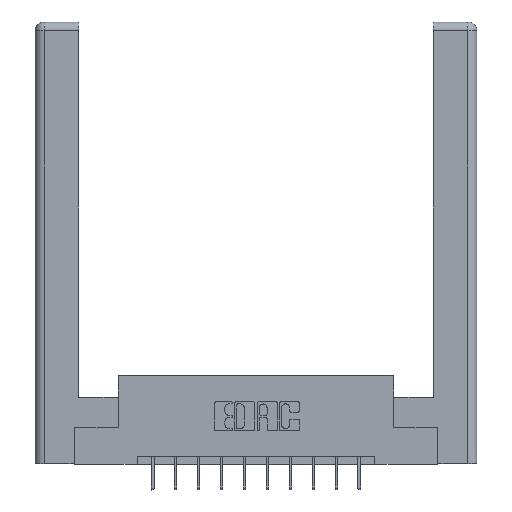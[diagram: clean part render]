
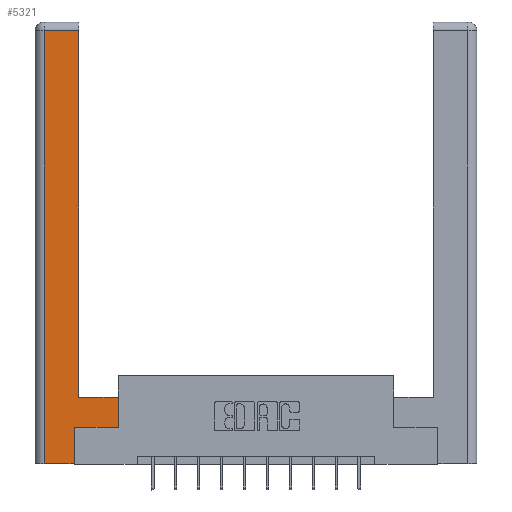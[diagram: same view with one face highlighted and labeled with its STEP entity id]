
A CAD part, top view. The second image highlights one B-rep face of the part: STEP entity #5321.
In plain terms, the highlighted planar face has unit normal (0, 0, 1).
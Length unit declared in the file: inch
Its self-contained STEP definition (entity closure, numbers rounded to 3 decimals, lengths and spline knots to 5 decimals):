
#81 = CARTESIAN_POINT ( 'NONE',  ( 0.0615, 2.94, 0. ) ) ;
#322 = CARTESIAN_POINT ( 'NONE',  ( 0., 0., 0. ) ) ;
#514 = DIRECTION ( 'NONE',  ( -1., 0., 0. ) ) ;
#683 = VERTEX_POINT ( 'NONE', #6908 ) ;
#721 = EDGE_CURVE ( 'NONE', #13895, #5554, #6565, .T. ) ;
#942 = EDGE_CURVE ( 'NONE', #5554, #4431, #7962, .T. ) ;
#1258 = LINE ( 'NONE', #3772, #2518 ) ;
#1772 = VECTOR ( 'NONE', #5712, 39.37008 ) ;
#1899 = VECTOR ( 'NONE', #7273, 39.37008 ) ;
#2169 = DIRECTION ( 'NONE',  ( 1., 0., 0. ) ) ;
#2438 = LINE ( 'NONE', #12914, #1899 ) ;
#2518 = VECTOR ( 'NONE', #514, 39.37008 ) ;
#2684 = CARTESIAN_POINT ( 'NONE',  ( 0.0615, 0., 0. ) ) ;
#2785 = DIRECTION ( 'NONE',  ( 0., -1., 0. ) ) ;
#3772 = CARTESIAN_POINT ( 'NONE',  ( 0.295, 0.45, 0. ) ) ;
#4431 = VERTEX_POINT ( 'NONE', #6519 ) ;
#4439 = CARTESIAN_POINT ( 'NONE',  ( 0.295, 0.45, 0. ) ) ;
#4937 = VECTOR ( 'NONE', #2785, 39.37008 ) ;
#4984 = VECTOR ( 'NONE', #2169, 39.37008 ) ;
#5105 = AXIS2_PLACEMENT_3D ( 'NONE', #322, #13936, #8277 ) ;
#5164 = LINE ( 'NONE', #11213, #9374 ) ;
#5321 = ADVANCED_FACE ( 'NONE', ( #13509 ), #11522, .F. ) ;
#5554 = VERTEX_POINT ( 'NONE', #5668 ) ;
#5594 = CARTESIAN_POINT ( 'NONE',  ( 0.265, 0.245, 0. ) ) ;
#5668 = CARTESIAN_POINT ( 'NONE',  ( 0.0615, 2.94, 0. ) ) ;
#5712 = DIRECTION ( 'NONE',  ( -1., 0., 0. ) ) ;
#5804 = VERTEX_POINT ( 'NONE', #14568 ) ;
#5915 = DIRECTION ( 'NONE',  ( 0., 1., 0. ) ) ;
#5949 = DIRECTION ( 'NONE',  ( 0., 1., 0. ) ) ;
#5997 = CARTESIAN_POINT ( 'NONE',  ( 0.295, 3., 0. ) ) ;
#6054 = VECTOR ( 'NONE', #5949, 39.37008 ) ;
#6519 = CARTESIAN_POINT ( 'NONE',  ( 0.0615, 0., 0. ) ) ;
#6565 = LINE ( 'NONE', #81, #1772 ) ;
#6908 = CARTESIAN_POINT ( 'NONE',  ( 0.565, 0.245, 0. ) ) ;
#7014 = CARTESIAN_POINT ( 'NONE',  ( 0.265, 0., 0. ) ) ;
#7174 = EDGE_CURVE ( 'NONE', #11089, #683, #7673, .T. ) ;
#7273 = DIRECTION ( 'NONE',  ( 0., 1., 0. ) ) ;
#7673 = LINE ( 'NONE', #13566, #4984 ) ;
#7681 = ORIENTED_EDGE ( 'NONE', *, *, #9911, .T. ) ;
#7861 = DIRECTION ( 'NONE',  ( 1., 0., 0. ) ) ;
#7962 = LINE ( 'NONE', #2684, #4937 ) ;
#8277 = DIRECTION ( 'NONE',  ( -1., 0., 0. ) ) ;
#8485 = VERTEX_POINT ( 'NONE', #4439 ) ;
#9306 = CARTESIAN_POINT ( 'NONE',  ( 0.565, 0.45, 0. ) ) ;
#9361 = EDGE_LOOP ( 'NONE', ( #11733, #12930, #11524, #13166, #10233, #10657, #14074, #7681 ) ) ;
#9374 = VECTOR ( 'NONE', #7861, 39.37008 ) ;
#9810 = VERTEX_POINT ( 'NONE', #7014 ) ;
#9844 = EDGE_CURVE ( 'NONE', #8485, #13895, #14343, .T. ) ;
#9911 = EDGE_CURVE ( 'NONE', #5804, #8485, #1258, .T. ) ;
#10233 = ORIENTED_EDGE ( 'NONE', *, *, #12101, .T. ) ;
#10657 = ORIENTED_EDGE ( 'NONE', *, *, #7174, .T. ) ;
#10757 = CARTESIAN_POINT ( 'NONE',  ( 0.295, 2.94, 0. ) ) ;
#11089 = VERTEX_POINT ( 'NONE', #5594 ) ;
#11213 = CARTESIAN_POINT ( 'NONE',  ( 0.265, 0., 0. ) ) ;
#11522 = PLANE ( 'NONE',  #5105 ) ;
#11524 = ORIENTED_EDGE ( 'NONE', *, *, #942, .T. ) ;
#11733 = ORIENTED_EDGE ( 'NONE', *, *, #9844, .T. ) ;
#12008 = EDGE_CURVE ( 'NONE', #683, #5804, #13574, .T. ) ;
#12101 = EDGE_CURVE ( 'NONE', #9810, #11089, #2438, .T. ) ;
#12914 = CARTESIAN_POINT ( 'NONE',  ( 0.265, 0.245, 0. ) ) ;
#12930 = ORIENTED_EDGE ( 'NONE', *, *, #721, .T. ) ;
#13166 = ORIENTED_EDGE ( 'NONE', *, *, #13562, .T. ) ;
#13233 = VECTOR ( 'NONE', #5915, 39.37008 ) ;
#13509 = FACE_OUTER_BOUND ( 'NONE', #9361, .T. ) ;
#13562 = EDGE_CURVE ( 'NONE', #4431, #9810, #5164, .T. ) ;
#13566 = CARTESIAN_POINT ( 'NONE',  ( 0.565, 0.245, 0. ) ) ;
#13574 = LINE ( 'NONE', #9306, #13233 ) ;
#13895 = VERTEX_POINT ( 'NONE', #10757 ) ;
#13936 = DIRECTION ( 'NONE',  ( 0., 0., -1. ) ) ;
#14074 = ORIENTED_EDGE ( 'NONE', *, *, #12008, .T. ) ;
#14343 = LINE ( 'NONE', #5997, #6054 ) ;
#14568 = CARTESIAN_POINT ( 'NONE',  ( 0.565, 0.45, 0. ) ) ;
